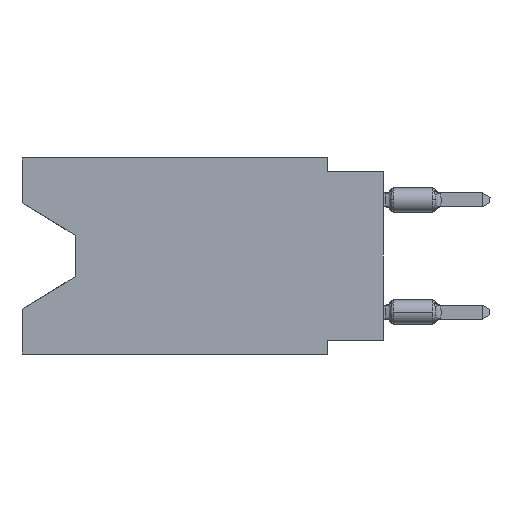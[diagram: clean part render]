
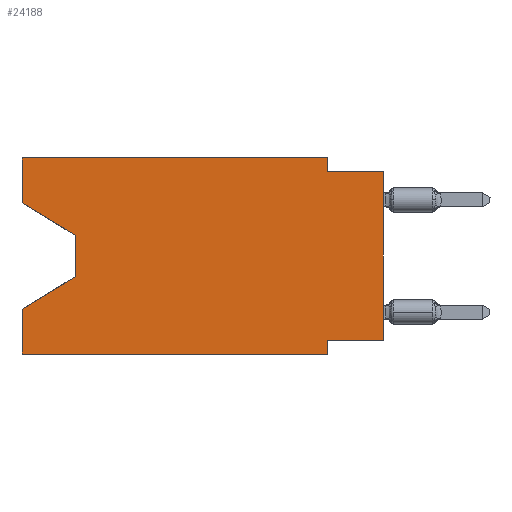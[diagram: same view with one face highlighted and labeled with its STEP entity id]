
A CAD part, left-side view. The second image highlights one B-rep face of the part: STEP entity #24188.
In plain terms, the highlighted planar face has unit normal (-1, 0, 0).
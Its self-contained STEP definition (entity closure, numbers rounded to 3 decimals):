
#161 = AXIS2_PLACEMENT_3D ( 'NONE', #43234, #16936, #47944 ) ;
#785 = EDGE_CURVE ( 'NONE', #15923, #52309, #53165, .T. ) ;
#1485 = VERTEX_POINT ( 'NONE', #44642 ) ;
#1846 = LINE ( 'NONE', #20136, #21131 ) ;
#2386 = VECTOR ( 'NONE', #42914, 1000. ) ;
#2684 = EDGE_CURVE ( 'NONE', #33046, #49538, #32306, .T. ) ;
#3398 = EDGE_CURVE ( 'NONE', #56456, #15328, #7142, .T. ) ;
#3928 = PLANE ( 'NONE',  #161 ) ;
#4499 = EDGE_CURVE ( 'NONE', #58095, #49538, #46134, .T. ) ;
#4856 = DIRECTION ( 'NONE',  ( 0., 0., 1. ) ) ;
#6982 = CARTESIAN_POINT ( 'NONE',  ( 0., 2.54, -8.255 ) ) ;
#7142 = LINE ( 'NONE', #52580, #37559 ) ;
#7464 = DIRECTION ( 'NONE',  ( 0., 1., 0. ) ) ;
#7909 = EDGE_CURVE ( 'NONE', #15328, #58095, #8835, .T. ) ;
#8835 = LINE ( 'NONE', #26848, #49216 ) ;
#10747 = EDGE_LOOP ( 'NONE', ( #10847, #34999, #24950, #49298, #38815, #15534, #44892, #50115, #41034, #26018, #18806, #46340 ) ) ;
#10847 = ORIENTED_EDGE ( 'NONE', *, *, #30532, .T. ) ;
#10997 = DIRECTION ( 'NONE',  ( 0., -1., 0. ) ) ;
#11120 = CARTESIAN_POINT ( 'NONE',  ( 0., 0., -8.255 ) ) ;
#11180 = CARTESIAN_POINT ( 'NONE',  ( 0., 13.97, -3.505 ) ) ;
#11299 = DIRECTION ( 'NONE',  ( 0., 0., -1. ) ) ;
#11906 = LINE ( 'NONE', #39350, #19993 ) ;
#13143 = VECTOR ( 'NONE', #10997, 1000. ) ;
#14278 = CARTESIAN_POINT ( 'NONE',  ( 0., 2.54, 0. ) ) ;
#14424 = LINE ( 'NONE', #36285, #57988 ) ;
#15328 = VERTEX_POINT ( 'NONE', #14278 ) ;
#15534 = ORIENTED_EDGE ( 'NONE', *, *, #42054, .F. ) ;
#15883 = DIRECTION ( 'NONE',  ( 0., 0.855, -0.519 ) ) ;
#15923 = VERTEX_POINT ( 'NONE', #43404 ) ;
#16272 = DIRECTION ( 'NONE',  ( 0., -1., 0. ) ) ;
#16903 = LINE ( 'NONE', #20468, #2386 ) ;
#16936 = DIRECTION ( 'NONE',  ( 1., 0., 0. ) ) ;
#17415 = DIRECTION ( 'NONE',  ( 0., 0., -1. ) ) ;
#18806 = ORIENTED_EDGE ( 'NONE', *, *, #3398, .F. ) ;
#19993 = VECTOR ( 'NONE', #7464, 1000. ) ;
#20017 = EDGE_CURVE ( 'NONE', #52055, #56456, #38544, .T. ) ;
#20136 = CARTESIAN_POINT ( 'NONE',  ( 0., 2.54, -8.89 ) ) ;
#20468 = CARTESIAN_POINT ( 'NONE',  ( 0., 16.383, -2.038 ) ) ;
#21131 = VECTOR ( 'NONE', #11299, 1000. ) ;
#24188 = ADVANCED_FACE ( 'NONE', ( #47663 ), #3928, .F. ) ;
#24330 = CARTESIAN_POINT ( 'NONE',  ( 0., 16.383, -6.852 ) ) ;
#24950 = ORIENTED_EDGE ( 'NONE', *, *, #35508, .T. ) ;
#24955 = DIRECTION ( 'NONE',  ( 0., 0., 1. ) ) ;
#26002 = VERTEX_POINT ( 'NONE', #24330 ) ;
#26018 = ORIENTED_EDGE ( 'NONE', *, *, #7909, .F. ) ;
#26848 = CARTESIAN_POINT ( 'NONE',  ( 0., 2.54, 0. ) ) ;
#26854 = LINE ( 'NONE', #54299, #44823 ) ;
#27008 = VERTEX_POINT ( 'NONE', #6982 ) ;
#27954 = VECTOR ( 'NONE', #48742, 1000. ) ;
#28422 = CARTESIAN_POINT ( 'NONE',  ( 0., 16.383, 0. ) ) ;
#30355 = CARTESIAN_POINT ( 'NONE',  ( 0., 0., -0.635 ) ) ;
#30532 = EDGE_CURVE ( 'NONE', #52055, #31356, #16903, .T. ) ;
#31083 = EDGE_CURVE ( 'NONE', #15923, #26002, #26854, .T. ) ;
#31356 = VERTEX_POINT ( 'NONE', #11180 ) ;
#32306 = LINE ( 'NONE', #35868, #38576 ) ;
#33046 = VERTEX_POINT ( 'NONE', #11120 ) ;
#33234 = EDGE_CURVE ( 'NONE', #33046, #27008, #11906, .T. ) ;
#34466 = CARTESIAN_POINT ( 'NONE',  ( 0., 2.54, -8.89 ) ) ;
#34603 = CARTESIAN_POINT ( 'NONE',  ( 0., 16.383, -2.038 ) ) ;
#34999 = ORIENTED_EDGE ( 'NONE', *, *, #47101, .T. ) ;
#35508 = EDGE_CURVE ( 'NONE', #1485, #26002, #38328, .T. ) ;
#35868 = CARTESIAN_POINT ( 'NONE',  ( 0., 0., 0. ) ) ;
#36285 = CARTESIAN_POINT ( 'NONE',  ( 0., 13.97, -3.505 ) ) ;
#36573 = DIRECTION ( 'NONE',  ( 0., 0., -1. ) ) ;
#37559 = VECTOR ( 'NONE', #16272, 1000. ) ;
#38247 = CARTESIAN_POINT ( 'NONE',  ( 0., 16.383, 0. ) ) ;
#38328 = LINE ( 'NONE', #56325, #43643 ) ;
#38544 = LINE ( 'NONE', #38247, #39287 ) ;
#38576 = VECTOR ( 'NONE', #4856, 1000. ) ;
#38815 = ORIENTED_EDGE ( 'NONE', *, *, #785, .T. ) ;
#39287 = VECTOR ( 'NONE', #24955, 1000. ) ;
#39350 = CARTESIAN_POINT ( 'NONE',  ( 0., 0., -8.255 ) ) ;
#40741 = CARTESIAN_POINT ( 'NONE',  ( 0., 2.54, -0.635 ) ) ;
#41034 = ORIENTED_EDGE ( 'NONE', *, *, #4499, .F. ) ;
#42054 = EDGE_CURVE ( 'NONE', #27008, #52309, #1846, .T. ) ;
#42914 = DIRECTION ( 'NONE',  ( 0., -0.855, -0.519 ) ) ;
#43234 = CARTESIAN_POINT ( 'NONE',  ( 0., 16.383, 0. ) ) ;
#43404 = CARTESIAN_POINT ( 'NONE',  ( 0., 16.383, -8.89 ) ) ;
#43643 = VECTOR ( 'NONE', #15883, 1000. ) ;
#44642 = CARTESIAN_POINT ( 'NONE',  ( 0., 13.97, -5.385 ) ) ;
#44823 = VECTOR ( 'NONE', #44871, 1000. ) ;
#44871 = DIRECTION ( 'NONE',  ( 0., 0., 1. ) ) ;
#44892 = ORIENTED_EDGE ( 'NONE', *, *, #33234, .F. ) ;
#46134 = LINE ( 'NONE', #46426, #13143 ) ;
#46340 = ORIENTED_EDGE ( 'NONE', *, *, #20017, .F. ) ;
#46426 = CARTESIAN_POINT ( 'NONE',  ( 0., 0., -0.635 ) ) ;
#47101 = EDGE_CURVE ( 'NONE', #31356, #1485, #14424, .T. ) ;
#47663 = FACE_OUTER_BOUND ( 'NONE', #10747, .T. ) ;
#47944 = DIRECTION ( 'NONE',  ( 0., 0., -1. ) ) ;
#48159 = CARTESIAN_POINT ( 'NONE',  ( 0., 16.383, -8.89 ) ) ;
#48742 = DIRECTION ( 'NONE',  ( 0., -1., 0. ) ) ;
#49216 = VECTOR ( 'NONE', #17415, 1000. ) ;
#49298 = ORIENTED_EDGE ( 'NONE', *, *, #31083, .F. ) ;
#49538 = VERTEX_POINT ( 'NONE', #30355 ) ;
#50115 = ORIENTED_EDGE ( 'NONE', *, *, #2684, .T. ) ;
#52055 = VERTEX_POINT ( 'NONE', #34603 ) ;
#52309 = VERTEX_POINT ( 'NONE', #34466 ) ;
#52580 = CARTESIAN_POINT ( 'NONE',  ( 0., 16.383, 0. ) ) ;
#53165 = LINE ( 'NONE', #48159, #27954 ) ;
#54299 = CARTESIAN_POINT ( 'NONE',  ( 0., 16.383, 0. ) ) ;
#56325 = CARTESIAN_POINT ( 'NONE',  ( 0., 13.97, -5.385 ) ) ;
#56456 = VERTEX_POINT ( 'NONE', #28422 ) ;
#57988 = VECTOR ( 'NONE', #36573, 1000. ) ;
#58095 = VERTEX_POINT ( 'NONE', #40741 ) ;
